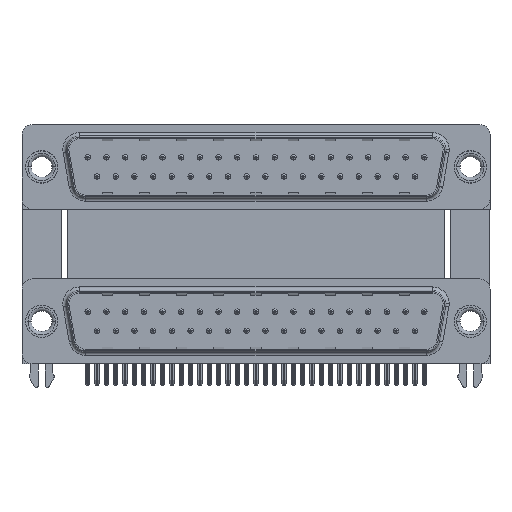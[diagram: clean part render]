
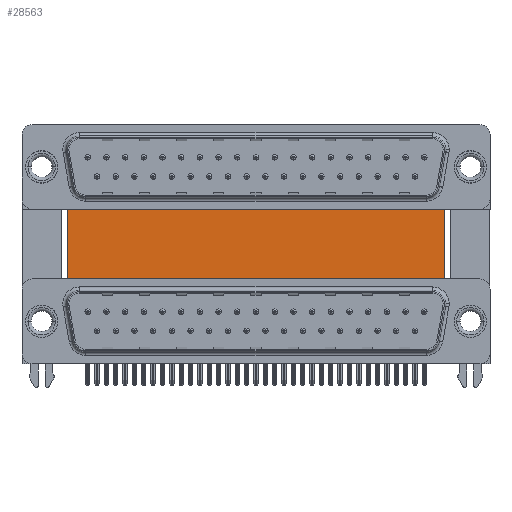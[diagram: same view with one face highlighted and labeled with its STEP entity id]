
A CAD part, top view. The second image highlights one B-rep face of the part: STEP entity #28563.
In plain terms, the highlighted planar face has unit normal (0, 0, 1).
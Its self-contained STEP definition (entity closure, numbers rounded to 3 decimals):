
#1965 = VECTOR ( 'NONE', #41806, 1000. ) ;
#2008 = DIRECTION ( 'NONE',  ( 1., 0., 0. ) ) ;
#2273 = LINE ( 'NONE', #10674, #11489 ) ;
#5814 = VERTEX_POINT ( 'NONE', #29102 ) ;
#6997 = EDGE_CURVE ( 'NONE', #5814, #26609, #2273, .T. ) ;
#8218 = EDGE_CURVE ( 'NONE', #35082, #47235, #33835, .T. ) ;
#9483 = EDGE_LOOP ( 'NONE', ( #10206, #34678, #12898, #11699 ) ) ;
#10206 = ORIENTED_EDGE ( 'NONE', *, *, #6997, .T. ) ;
#10674 = CARTESIAN_POINT ( 'NONE',  ( 3.79, -3.735, -12. ) ) ;
#11489 = VECTOR ( 'NONE', #2008, 1000. ) ;
#11699 = ORIENTED_EDGE ( 'NONE', *, *, #21063, .T. ) ;
#12898 = ORIENTED_EDGE ( 'NONE', *, *, #8218, .F. ) ;
#14729 = LINE ( 'NONE', #26933, #22213 ) ;
#21063 = EDGE_CURVE ( 'NONE', #35082, #5814, #14729, .T. ) ;
#22036 = FACE_OUTER_BOUND ( 'NONE', #9483, .T. ) ;
#22213 = VECTOR ( 'NONE', #26422, 1000. ) ;
#26095 = DIRECTION ( 'NONE',  ( 0., 0., -1. ) ) ;
#26422 = DIRECTION ( 'NONE',  ( 0., -1., 0. ) ) ;
#26609 = VERTEX_POINT ( 'NONE', #29945 ) ;
#26933 = CARTESIAN_POINT ( 'NONE',  ( 3.79, 16.585, -12. ) ) ;
#28538 = CARTESIAN_POINT ( 'NONE',  ( 59.71, 16.585, -12. ) ) ;
#28563 = ADVANCED_FACE ( 'NONE', ( #22036 ), #29933, .F. ) ;
#29102 = CARTESIAN_POINT ( 'NONE',  ( 3.79, -3.735, -12. ) ) ;
#29864 = LINE ( 'NONE', #30626, #1965 ) ;
#29933 = PLANE ( 'NONE',  #38152 ) ;
#29945 = CARTESIAN_POINT ( 'NONE',  ( 59.71, -3.735, -12. ) ) ;
#30014 = DIRECTION ( 'NONE',  ( 1., 0., 0. ) ) ;
#30626 = CARTESIAN_POINT ( 'NONE',  ( 59.71, 16.585, -12. ) ) ;
#33265 = CARTESIAN_POINT ( 'NONE',  ( 3.79, 16.585, -12. ) ) ;
#33835 = LINE ( 'NONE', #45538, #33965 ) ;
#33965 = VECTOR ( 'NONE', #30014, 1000. ) ;
#34678 = ORIENTED_EDGE ( 'NONE', *, *, #35675, .F. ) ;
#35082 = VERTEX_POINT ( 'NONE', #37749 ) ;
#35675 = EDGE_CURVE ( 'NONE', #47235, #26609, #29864, .T. ) ;
#37749 = CARTESIAN_POINT ( 'NONE',  ( 3.79, 16.585, -12. ) ) ;
#38152 = AXIS2_PLACEMENT_3D ( 'NONE', #33265, #26095, #45451 ) ;
#41806 = DIRECTION ( 'NONE',  ( 0., -1., 0. ) ) ;
#45451 = DIRECTION ( 'NONE',  ( -1., 0., 0. ) ) ;
#45538 = CARTESIAN_POINT ( 'NONE',  ( 3.79, 16.585, -12. ) ) ;
#47235 = VERTEX_POINT ( 'NONE', #28538 ) ;
